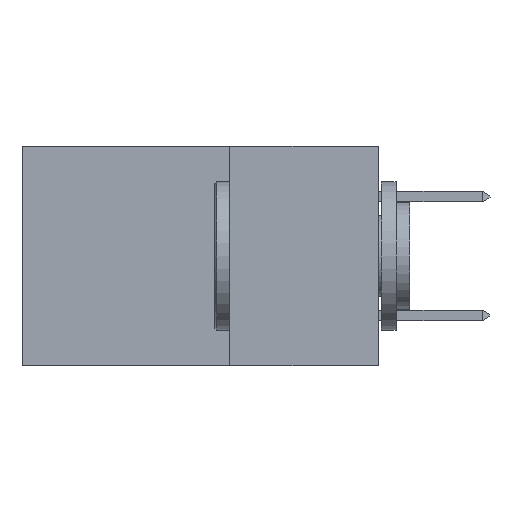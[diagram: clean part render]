
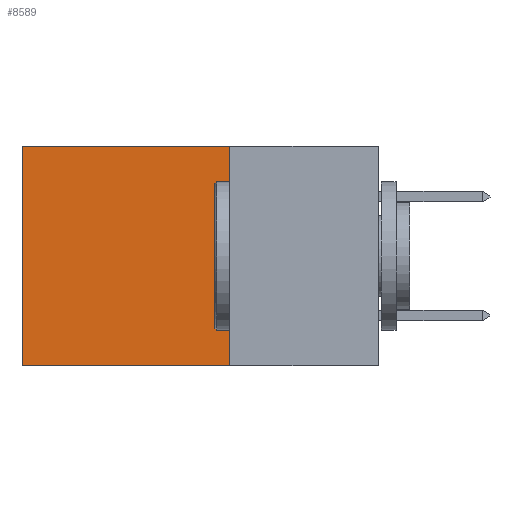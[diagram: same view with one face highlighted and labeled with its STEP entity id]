
A CAD part, left-side view. The second image highlights one B-rep face of the part: STEP entity #8589.
In plain terms, the highlighted planar face has unit normal (-1, 0, 0).
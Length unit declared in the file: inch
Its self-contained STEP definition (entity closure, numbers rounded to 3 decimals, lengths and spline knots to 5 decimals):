
#156 = VECTOR ( 'NONE', #19674, 39.37008 ) ;
#318 = ORIENTED_EDGE ( 'NONE', *, *, #14112, .F. ) ;
#759 = FACE_OUTER_BOUND ( 'NONE', #15756, .T. ) ;
#829 = CARTESIAN_POINT ( 'NONE',  ( 0.298, 0.6, -0.37 ) ) ;
#1021 = CARTESIAN_POINT ( 'NONE',  ( 0.298, 0.25, 0. ) ) ;
#2682 = DIRECTION ( 'NONE',  ( 0., 0., -1. ) ) ;
#4040 = CARTESIAN_POINT ( 'NONE',  ( 0.298, 0.25, -0.37 ) ) ;
#4342 = CARTESIAN_POINT ( 'NONE',  ( 0.298, 0.25, -0.37 ) ) ;
#5925 = VERTEX_POINT ( 'NONE', #18328 ) ;
#7009 = ORIENTED_EDGE ( 'NONE', *, *, #18007, .T. ) ;
#8452 = CARTESIAN_POINT ( 'NONE',  ( 0.298, 0.25, 0. ) ) ;
#8589 = ADVANCED_FACE ( 'NONE', ( #759 ), #10864, .F. ) ;
#8698 = LINE ( 'NONE', #4342, #12467 ) ;
#10864 = PLANE ( 'NONE',  #14519 ) ;
#11656 = CARTESIAN_POINT ( 'NONE',  ( 0.298, 0.25, 0. ) ) ;
#11932 = CARTESIAN_POINT ( 'NONE',  ( 0.298, 0.6, 0. ) ) ;
#12008 = DIRECTION ( 'NONE',  ( 0., 0., -1. ) ) ;
#12282 = ORIENTED_EDGE ( 'NONE', *, *, #20152, .F. ) ;
#12467 = VECTOR ( 'NONE', #14084, 39.37008 ) ;
#12498 = DIRECTION ( 'NONE',  ( 1., 0., 0. ) ) ;
#13459 = CARTESIAN_POINT ( 'NONE',  ( 0.298, 0.25, 0. ) ) ;
#14084 = DIRECTION ( 'NONE',  ( 0., 1., 0. ) ) ;
#14112 = EDGE_CURVE ( 'NONE', #20389, #15982, #8698, .T. ) ;
#14519 = AXIS2_PLACEMENT_3D ( 'NONE', #1021, #12498, #2682 ) ;
#14871 = DIRECTION ( 'NONE',  ( 0., 1., 0. ) ) ;
#15413 = VECTOR ( 'NONE', #12008, 39.37008 ) ;
#15756 = EDGE_LOOP ( 'NONE', ( #20766, #318, #12282, #7009 ) ) ;
#15809 = VERTEX_POINT ( 'NONE', #13459 ) ;
#15982 = VERTEX_POINT ( 'NONE', #829 ) ;
#16199 = LINE ( 'NONE', #11656, #19867 ) ;
#17107 = LINE ( 'NONE', #8452, #156 ) ;
#18007 = EDGE_CURVE ( 'NONE', #15809, #5925, #16199, .T. ) ;
#18121 = EDGE_CURVE ( 'NONE', #5925, #15982, #19617, .T. ) ;
#18328 = CARTESIAN_POINT ( 'NONE',  ( 0.298, 0.6, 0. ) ) ;
#19617 = LINE ( 'NONE', #11932, #15413 ) ;
#19674 = DIRECTION ( 'NONE',  ( 0., 0., -1. ) ) ;
#19867 = VECTOR ( 'NONE', #14871, 39.37008 ) ;
#20152 = EDGE_CURVE ( 'NONE', #15809, #20389, #17107, .T. ) ;
#20389 = VERTEX_POINT ( 'NONE', #4040 ) ;
#20766 = ORIENTED_EDGE ( 'NONE', *, *, #18121, .T. ) ;
